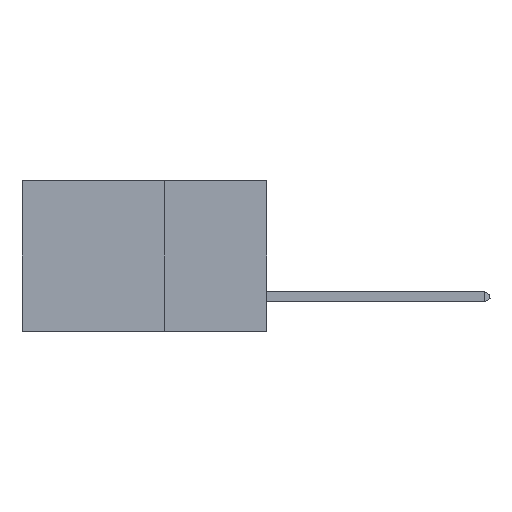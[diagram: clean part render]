
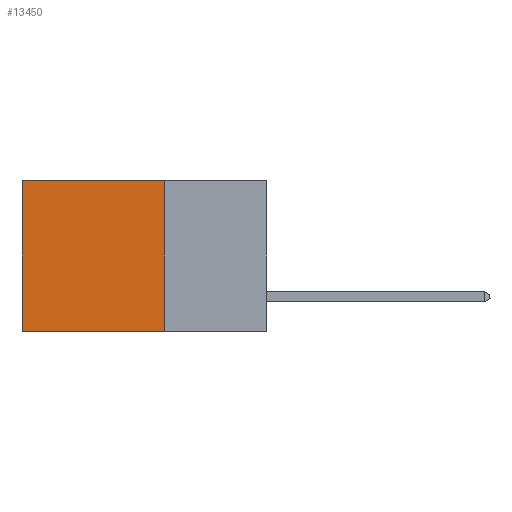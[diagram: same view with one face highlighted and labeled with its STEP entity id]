
A CAD part, left-side view. The second image highlights one B-rep face of the part: STEP entity #13450.
In plain terms, the highlighted planar face has unit normal (-1, 0, 0).
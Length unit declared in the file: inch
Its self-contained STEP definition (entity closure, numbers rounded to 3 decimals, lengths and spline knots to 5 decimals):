
#441 = EDGE_CURVE ( 'NONE', #8621, #9181, #10458, .T. ) ;
#496 = VERTEX_POINT ( 'NONE', #14062 ) ;
#1093 = VECTOR ( 'NONE', #10530, 39.37008 ) ;
#1293 = VECTOR ( 'NONE', #12962, 39.37008 ) ;
#1378 = LINE ( 'NONE', #7411, #11038 ) ;
#1411 = CARTESIAN_POINT ( 'NONE',  ( 0.2875, 0.6, 0. ) ) ;
#1979 = PLANE ( 'NONE',  #11472 ) ;
#2146 = ORIENTED_EDGE ( 'NONE', *, *, #14047, .T. ) ;
#2309 = VECTOR ( 'NONE', #3731, 39.37008 ) ;
#3731 = DIRECTION ( 'NONE',  ( 0., 1., 0. ) ) ;
#4820 = CARTESIAN_POINT ( 'NONE',  ( 0.2875, 0.6, 0. ) ) ;
#5195 = CARTESIAN_POINT ( 'NONE',  ( 0.2875, 0.25, 0. ) ) ;
#6471 = EDGE_CURVE ( 'NONE', #9181, #496, #8667, .T. ) ;
#7411 = CARTESIAN_POINT ( 'NONE',  ( 0.2875, 0.25, 0. ) ) ;
#7683 = CARTESIAN_POINT ( 'NONE',  ( 0.2875, 0.25, 0. ) ) ;
#7955 = ORIENTED_EDGE ( 'NONE', *, *, #6471, .F. ) ;
#8551 = CARTESIAN_POINT ( 'NONE',  ( 0.2875, 0.25, 0. ) ) ;
#8621 = VERTEX_POINT ( 'NONE', #7683 ) ;
#8667 = LINE ( 'NONE', #11119, #2309 ) ;
#8760 = ORIENTED_EDGE ( 'NONE', *, *, #10632, .T. ) ;
#9181 = VERTEX_POINT ( 'NONE', #10521 ) ;
#9672 = DIRECTION ( 'NONE',  ( 0., 0., -1. ) ) ;
#9908 = LINE ( 'NONE', #4820, #1093 ) ;
#10458 = LINE ( 'NONE', #5195, #1293 ) ;
#10521 = CARTESIAN_POINT ( 'NONE',  ( 0.2875, 0.25, -0.37 ) ) ;
#10530 = DIRECTION ( 'NONE',  ( 0., 0., -1. ) ) ;
#10632 = EDGE_CURVE ( 'NONE', #13784, #496, #9908, .T. ) ;
#11038 = VECTOR ( 'NONE', #11894, 39.37008 ) ;
#11044 = ORIENTED_EDGE ( 'NONE', *, *, #441, .F. ) ;
#11119 = CARTESIAN_POINT ( 'NONE',  ( 0.2875, 0.25, -0.37 ) ) ;
#11472 = AXIS2_PLACEMENT_3D ( 'NONE', #8551, #11818, #9672 ) ;
#11818 = DIRECTION ( 'NONE',  ( 1., 0., 0. ) ) ;
#11894 = DIRECTION ( 'NONE',  ( 0., 1., 0. ) ) ;
#12236 = FACE_OUTER_BOUND ( 'NONE', #12710, .T. ) ;
#12710 = EDGE_LOOP ( 'NONE', ( #8760, #7955, #11044, #2146 ) ) ;
#12962 = DIRECTION ( 'NONE',  ( 0., 0., -1. ) ) ;
#13450 = ADVANCED_FACE ( 'NONE', ( #12236 ), #1979, .F. ) ;
#13784 = VERTEX_POINT ( 'NONE', #1411 ) ;
#14047 = EDGE_CURVE ( 'NONE', #8621, #13784, #1378, .T. ) ;
#14062 = CARTESIAN_POINT ( 'NONE',  ( 0.2875, 0.6, -0.37 ) ) ;
